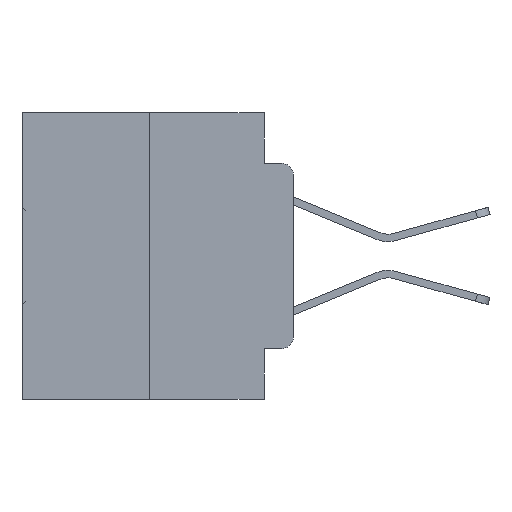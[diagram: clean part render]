
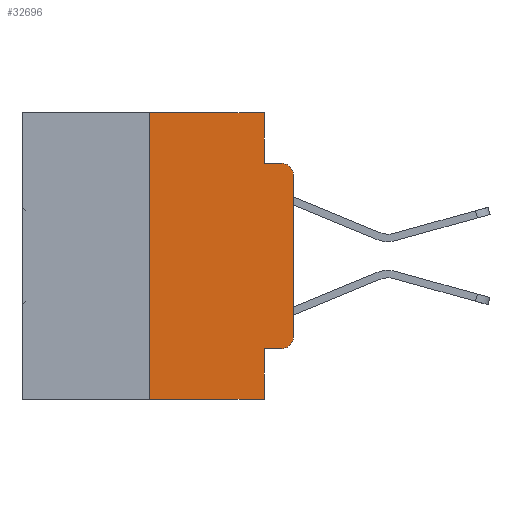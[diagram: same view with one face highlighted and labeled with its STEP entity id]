
A CAD part, left-side view. The second image highlights one B-rep face of the part: STEP entity #32696.
In plain terms, the highlighted planar face has unit normal (-1, 0, 0).
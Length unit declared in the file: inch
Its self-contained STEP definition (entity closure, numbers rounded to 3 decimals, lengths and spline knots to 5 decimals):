
#46 = DIRECTION ( 'NONE',  ( 0., 0., -1. ) ) ;
#448 = FACE_OUTER_BOUND ( 'NONE', #9728, .T. ) ;
#987 = CARTESIAN_POINT ( 'NONE',  ( 0., 0.051, -0.4115 ) ) ;
#1220 = CARTESIAN_POINT ( 'NONE',  ( 0., 0.25, -0.5 ) ) ;
#1426 = CARTESIAN_POINT ( 'NONE',  ( 0., 0.25, 0. ) ) ;
#1906 = AXIS2_PLACEMENT_3D ( 'NONE', #30494, #15399, #46 ) ;
#2151 = VERTEX_POINT ( 'NONE', #16538 ) ;
#2907 = ORIENTED_EDGE ( 'NONE', *, *, #26784, .F. ) ;
#2914 = ORIENTED_EDGE ( 'NONE', *, *, #28468, .F. ) ;
#2919 = LINE ( 'NONE', #25540, #8941 ) ;
#3367 = CARTESIAN_POINT ( 'NONE',  ( 0., 0., -0.1085 ) ) ;
#3649 = DIRECTION ( 'NONE',  ( 0., -1., 0. ) ) ;
#3668 = DIRECTION ( 'NONE',  ( 0., -1., 0. ) ) ;
#3816 = VERTEX_POINT ( 'NONE', #29984 ) ;
#3915 = DIRECTION ( 'NONE',  ( 0., 0., 1. ) ) ;
#4148 = EDGE_CURVE ( 'NONE', #27417, #31666, #21296, .T. ) ;
#4601 = EDGE_CURVE ( 'NONE', #28274, #3816, #22056, .T. ) ;
#5060 = VERTEX_POINT ( 'NONE', #19714 ) ;
#5453 = LINE ( 'NONE', #21417, #31447 ) ;
#5874 = EDGE_CURVE ( 'NONE', #31666, #30929, #28626, .T. ) ;
#7577 = EDGE_CURVE ( 'NONE', #13768, #30929, #16432, .T. ) ;
#7708 = ORIENTED_EDGE ( 'NONE', *, *, #12600, .T. ) ;
#7834 = VECTOR ( 'NONE', #11108, 39.37008 ) ;
#8278 = DIRECTION ( 'NONE',  ( 0., -1., 0. ) ) ;
#8503 = VECTOR ( 'NONE', #8278, 39.37008 ) ;
#8878 = PLANE ( 'NONE',  #22657 ) ;
#8941 = VECTOR ( 'NONE', #18041, 39.37008 ) ;
#9728 = EDGE_LOOP ( 'NONE', ( #7708, #24312, #29425, #23559, #20030, #2914, #14781, #2907, #15663, #22423 ) ) ;
#9812 = CARTESIAN_POINT ( 'NONE',  ( 0., 0.051, -0.0885 ) ) ;
#10159 = DIRECTION ( 'NONE',  ( -1., 0., 0. ) ) ;
#11108 = DIRECTION ( 'NONE',  ( 0., 0., -1. ) ) ;
#12600 = EDGE_CURVE ( 'NONE', #2151, #13768, #17267, .T. ) ;
#12916 = LINE ( 'NONE', #987, #25602 ) ;
#13427 = VERTEX_POINT ( 'NONE', #14680 ) ;
#13768 = VERTEX_POINT ( 'NONE', #3367 ) ;
#13904 = DIRECTION ( 'NONE',  ( 1., 0., 0. ) ) ;
#14680 = CARTESIAN_POINT ( 'NONE',  ( 0., 0.051, -0.4115 ) ) ;
#14781 = ORIENTED_EDGE ( 'NONE', *, *, #4601, .T. ) ;
#15102 = AXIS2_PLACEMENT_3D ( 'NONE', #25289, #10159, #27801 ) ;
#15399 = DIRECTION ( 'NONE',  ( -1., 0., 0. ) ) ;
#15663 = ORIENTED_EDGE ( 'NONE', *, *, #25111, .T. ) ;
#16432 = CIRCLE ( 'NONE', #15102, 0.02 ) ;
#16538 = CARTESIAN_POINT ( 'NONE',  ( 0., 0., -0.3915 ) ) ;
#17267 = LINE ( 'NONE', #26676, #29868 ) ;
#18041 = DIRECTION ( 'NONE',  ( 0., 0., -1. ) ) ;
#18360 = EDGE_CURVE ( 'NONE', #5060, #2151, #31818, .T. ) ;
#19714 = CARTESIAN_POINT ( 'NONE',  ( 0., 0.02, -0.4115 ) ) ;
#19845 = CARTESIAN_POINT ( 'NONE',  ( 0., 0.25, 0. ) ) ;
#20030 = ORIENTED_EDGE ( 'NONE', *, *, #32033, .F. ) ;
#20458 = VECTOR ( 'NONE', #25457, 39.37008 ) ;
#21296 = LINE ( 'NONE', #31250, #7834 ) ;
#21417 = CARTESIAN_POINT ( 'NONE',  ( 0., 0.473, 0. ) ) ;
#22056 = LINE ( 'NONE', #22828, #20458 ) ;
#22423 = ORIENTED_EDGE ( 'NONE', *, *, #18360, .T. ) ;
#22657 = AXIS2_PLACEMENT_3D ( 'NONE', #29034, #13904, #31542 ) ;
#22828 = CARTESIAN_POINT ( 'NONE',  ( 0., 0.473, -0.5 ) ) ;
#23559 = ORIENTED_EDGE ( 'NONE', *, *, #4148, .F. ) ;
#23990 = VERTEX_POINT ( 'NONE', #1426 ) ;
#24312 = ORIENTED_EDGE ( 'NONE', *, *, #7577, .T. ) ;
#25111 = EDGE_CURVE ( 'NONE', #13427, #5060, #12916, .T. ) ;
#25289 = CARTESIAN_POINT ( 'NONE',  ( 0., 0.02, -0.1085 ) ) ;
#25421 = VECTOR ( 'NONE', #27409, 39.37008 ) ;
#25457 = DIRECTION ( 'NONE',  ( 0., -1., 0. ) ) ;
#25540 = CARTESIAN_POINT ( 'NONE',  ( 0., 0.051, 0. ) ) ;
#25602 = VECTOR ( 'NONE', #3649, 39.37008 ) ;
#26194 = LINE ( 'NONE', #19845, #25421 ) ;
#26676 = CARTESIAN_POINT ( 'NONE',  ( 0., 0., 0. ) ) ;
#26784 = EDGE_CURVE ( 'NONE', #13427, #3816, #2919, .T. ) ;
#27131 = CARTESIAN_POINT ( 'NONE',  ( 0., 0.02, -0.0885 ) ) ;
#27409 = DIRECTION ( 'NONE',  ( 0., 0., 1. ) ) ;
#27417 = VERTEX_POINT ( 'NONE', #30518 ) ;
#27801 = DIRECTION ( 'NONE',  ( 0., 0., -1. ) ) ;
#28274 = VERTEX_POINT ( 'NONE', #1220 ) ;
#28468 = EDGE_CURVE ( 'NONE', #28274, #23990, #26194, .T. ) ;
#28626 = LINE ( 'NONE', #30950, #8503 ) ;
#29034 = CARTESIAN_POINT ( 'NONE',  ( 0., 0.473, 0. ) ) ;
#29425 = ORIENTED_EDGE ( 'NONE', *, *, #5874, .F. ) ;
#29868 = VECTOR ( 'NONE', #3915, 39.37008 ) ;
#29984 = CARTESIAN_POINT ( 'NONE',  ( 0., 0.051, -0.5 ) ) ;
#30494 = CARTESIAN_POINT ( 'NONE',  ( 0., 0.02, -0.3915 ) ) ;
#30518 = CARTESIAN_POINT ( 'NONE',  ( 0., 0.051, 0. ) ) ;
#30929 = VERTEX_POINT ( 'NONE', #27131 ) ;
#30950 = CARTESIAN_POINT ( 'NONE',  ( 0., 0.051, -0.0885 ) ) ;
#31250 = CARTESIAN_POINT ( 'NONE',  ( 0., 0.051, 0. ) ) ;
#31447 = VECTOR ( 'NONE', #3668, 39.37008 ) ;
#31542 = DIRECTION ( 'NONE',  ( 0., 0., -1. ) ) ;
#31666 = VERTEX_POINT ( 'NONE', #9812 ) ;
#31818 = CIRCLE ( 'NONE', #1906, 0.02 ) ;
#32033 = EDGE_CURVE ( 'NONE', #23990, #27417, #5453, .T. ) ;
#32696 = ADVANCED_FACE ( 'NONE', ( #448 ), #8878, .F. ) ;
